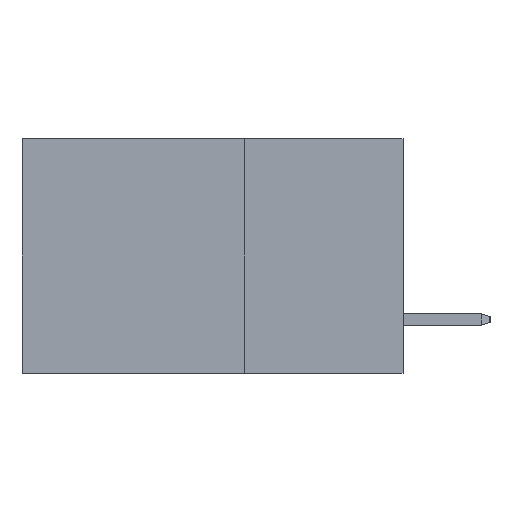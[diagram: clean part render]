
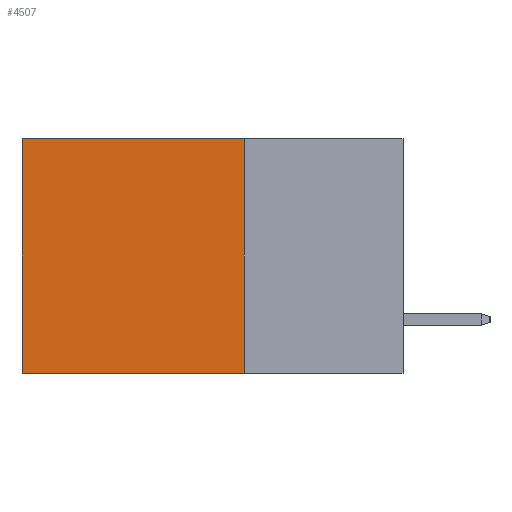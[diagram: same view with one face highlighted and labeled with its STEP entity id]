
A CAD part, left-side view. The second image highlights one B-rep face of the part: STEP entity #4507.
In plain terms, the highlighted planar face has unit normal (-1, 0, 0).
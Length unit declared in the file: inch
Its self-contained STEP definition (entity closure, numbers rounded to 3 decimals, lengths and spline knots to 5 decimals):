
#18 = DIRECTION ( 'NONE',  ( 0., 0., -1. ) ) ;
#35 = DIRECTION ( 'NONE',  ( 0., 0., -1. ) ) ;
#472 = DIRECTION ( 'NONE',  ( 0., 1., 0. ) ) ;
#595 = DIRECTION ( 'NONE',  ( 0., 0., -1. ) ) ;
#634 = DIRECTION ( 'NONE',  ( 0., 1., 0. ) ) ;
#679 = EDGE_CURVE ( 'NONE', #6065, #1696, #2855, .T. ) ;
#1454 = VERTEX_POINT ( 'NONE', #12066 ) ;
#1650 = LINE ( 'NONE', #11239, #2096 ) ;
#1652 = VECTOR ( 'NONE', #18, 39.37008 ) ;
#1688 = CARTESIAN_POINT ( 'NONE',  ( 0.2875, 0.25, 0. ) ) ;
#1696 = VERTEX_POINT ( 'NONE', #4000 ) ;
#2096 = VECTOR ( 'NONE', #595, 39.37008 ) ;
#2653 = ORIENTED_EDGE ( 'NONE', *, *, #7648, .T. ) ;
#2855 = LINE ( 'NONE', #5983, #5458 ) ;
#3235 = CARTESIAN_POINT ( 'NONE',  ( 0.2875, 0.25, 0. ) ) ;
#4000 = CARTESIAN_POINT ( 'NONE',  ( 0.2875, 0.6, -0.37 ) ) ;
#4304 = CARTESIAN_POINT ( 'NONE',  ( 0.2875, 0.6, 0. ) ) ;
#4480 = DIRECTION ( 'NONE',  ( 1., 0., 0. ) ) ;
#4507 = ADVANCED_FACE ( 'NONE', ( #12819 ), #12749, .F. ) ;
#5437 = LINE ( 'NONE', #11564, #1652 ) ;
#5458 = VECTOR ( 'NONE', #472, 39.37008 ) ;
#5983 = CARTESIAN_POINT ( 'NONE',  ( 0.2875, 0.25, -0.37 ) ) ;
#6065 = VERTEX_POINT ( 'NONE', #12063 ) ;
#6207 = LINE ( 'NONE', #1688, #9608 ) ;
#6644 = EDGE_CURVE ( 'NONE', #1454, #6741, #6207, .T. ) ;
#6741 = VERTEX_POINT ( 'NONE', #4304 ) ;
#6920 = AXIS2_PLACEMENT_3D ( 'NONE', #3235, #4480, #35 ) ;
#7648 = EDGE_CURVE ( 'NONE', #6741, #1696, #5437, .T. ) ;
#8199 = EDGE_CURVE ( 'NONE', #1454, #6065, #1650, .T. ) ;
#9608 = VECTOR ( 'NONE', #634, 39.37008 ) ;
#10289 = ORIENTED_EDGE ( 'NONE', *, *, #679, .F. ) ;
#11239 = CARTESIAN_POINT ( 'NONE',  ( 0.2875, 0.25, 0. ) ) ;
#11333 = ORIENTED_EDGE ( 'NONE', *, *, #6644, .T. ) ;
#11564 = CARTESIAN_POINT ( 'NONE',  ( 0.2875, 0.6, 0. ) ) ;
#11637 = ORIENTED_EDGE ( 'NONE', *, *, #8199, .F. ) ;
#12063 = CARTESIAN_POINT ( 'NONE',  ( 0.2875, 0.25, -0.37 ) ) ;
#12066 = CARTESIAN_POINT ( 'NONE',  ( 0.2875, 0.25, 0. ) ) ;
#12749 = PLANE ( 'NONE',  #6920 ) ;
#12819 = FACE_OUTER_BOUND ( 'NONE', #13536, .T. ) ;
#13536 = EDGE_LOOP ( 'NONE', ( #2653, #10289, #11637, #11333 ) ) ;
